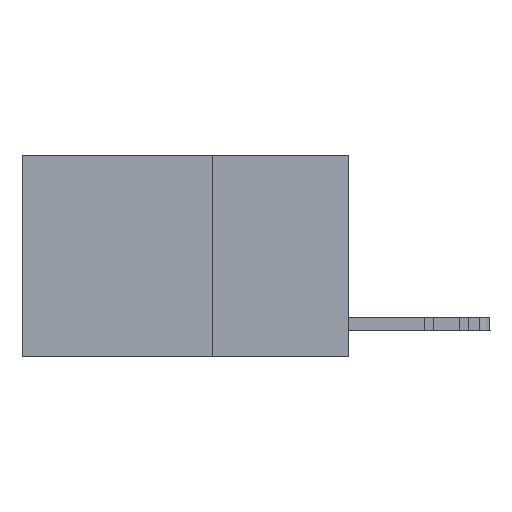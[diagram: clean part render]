
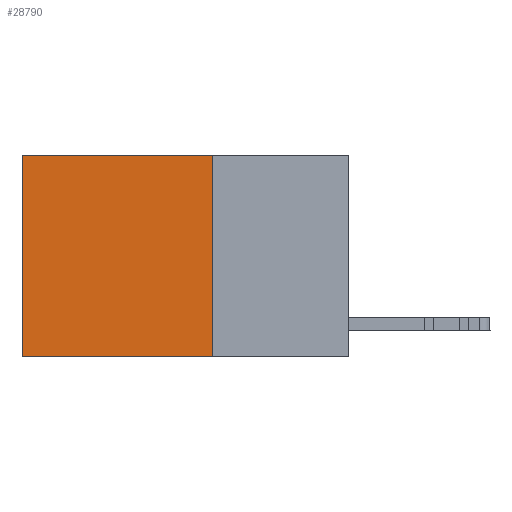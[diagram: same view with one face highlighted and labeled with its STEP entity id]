
A CAD part, left-side view. The second image highlights one B-rep face of the part: STEP entity #28790.
In plain terms, the highlighted planar face has unit normal (-1, 0, 0).
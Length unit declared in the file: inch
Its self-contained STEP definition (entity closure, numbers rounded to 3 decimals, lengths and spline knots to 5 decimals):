
#103 = ORIENTED_EDGE ( 'NONE', *, *, #633, .T. ) ;
#448 = DIRECTION ( 'NONE',  ( 0., 1., 0. ) ) ;
#541 = ORIENTED_EDGE ( 'NONE', *, *, #11264, .F. ) ;
#633 = EDGE_CURVE ( 'NONE', #23038, #9780, #24254, .T. ) ;
#1994 = EDGE_CURVE ( 'NONE', #9780, #25849, #20924, .T. ) ;
#2155 = CARTESIAN_POINT ( 'NONE',  ( 0.2625, 0.6, 0. ) ) ;
#3548 = CARTESIAN_POINT ( 'NONE',  ( 0.2625, 0.25, 0. ) ) ;
#4458 = LINE ( 'NONE', #21368, #22703 ) ;
#4504 = VECTOR ( 'NONE', #9198, 39.37008 ) ;
#6974 = EDGE_LOOP ( 'NONE', ( #17188, #19104, #541, #103 ) ) ;
#7539 = CARTESIAN_POINT ( 'NONE',  ( 0.2625, 0.25, 0. ) ) ;
#8679 = AXIS2_PLACEMENT_3D ( 'NONE', #7539, #18671, #25936 ) ;
#8702 = LINE ( 'NONE', #16171, #25755 ) ;
#8779 = CARTESIAN_POINT ( 'NONE',  ( 0.2625, 0.25, -0.37 ) ) ;
#9198 = DIRECTION ( 'NONE',  ( 0., 0., -1. ) ) ;
#9780 = VERTEX_POINT ( 'NONE', #19375 ) ;
#11127 = DIRECTION ( 'NONE',  ( 0., 0., -1. ) ) ;
#11264 = EDGE_CURVE ( 'NONE', #23038, #29344, #8702, .T. ) ;
#12851 = CARTESIAN_POINT ( 'NONE',  ( 0.2625, 0.6, -0.37 ) ) ;
#14123 = EDGE_CURVE ( 'NONE', #29344, #25849, #4458, .T. ) ;
#14230 = FACE_OUTER_BOUND ( 'NONE', #6974, .T. ) ;
#16171 = CARTESIAN_POINT ( 'NONE',  ( 0.2625, 0.25, 0. ) ) ;
#17188 = ORIENTED_EDGE ( 'NONE', *, *, #1994, .T. ) ;
#18543 = CARTESIAN_POINT ( 'NONE',  ( 0.2625, 0.25, 0. ) ) ;
#18671 = DIRECTION ( 'NONE',  ( 1., 0., 0. ) ) ;
#18811 = PLANE ( 'NONE',  #8679 ) ;
#19104 = ORIENTED_EDGE ( 'NONE', *, *, #14123, .F. ) ;
#19375 = CARTESIAN_POINT ( 'NONE',  ( 0.2625, 0.6, 0. ) ) ;
#20924 = LINE ( 'NONE', #2155, #4504 ) ;
#21368 = CARTESIAN_POINT ( 'NONE',  ( 0.2625, 0.25, -0.37 ) ) ;
#22703 = VECTOR ( 'NONE', #448, 39.37008 ) ;
#23038 = VERTEX_POINT ( 'NONE', #18543 ) ;
#23660 = VECTOR ( 'NONE', #24564, 39.37008 ) ;
#24254 = LINE ( 'NONE', #3548, #23660 ) ;
#24564 = DIRECTION ( 'NONE',  ( 0., 1., 0. ) ) ;
#25755 = VECTOR ( 'NONE', #11127, 39.37008 ) ;
#25849 = VERTEX_POINT ( 'NONE', #12851 ) ;
#25936 = DIRECTION ( 'NONE',  ( 0., 0., -1. ) ) ;
#28790 = ADVANCED_FACE ( 'NONE', ( #14230 ), #18811, .F. ) ;
#29344 = VERTEX_POINT ( 'NONE', #8779 ) ;
